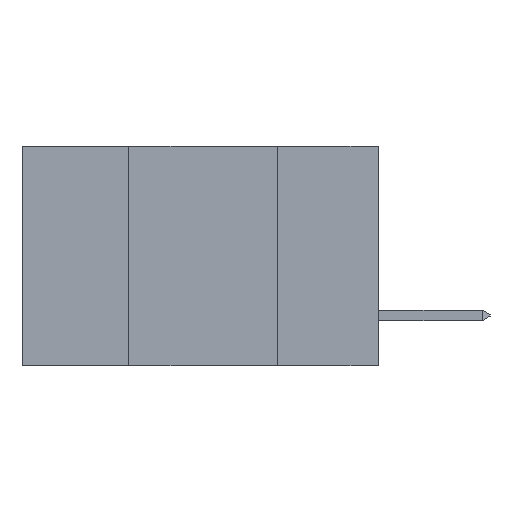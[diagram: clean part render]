
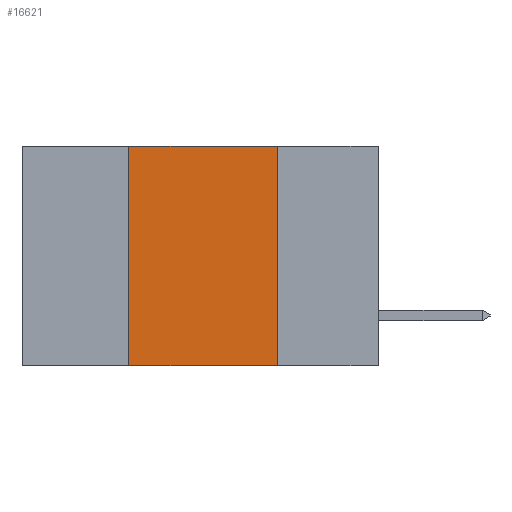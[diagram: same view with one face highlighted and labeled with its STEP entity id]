
A CAD part, left-side view. The second image highlights one B-rep face of the part: STEP entity #16621.
In plain terms, the highlighted planar face has unit normal (-1, 0, 0).
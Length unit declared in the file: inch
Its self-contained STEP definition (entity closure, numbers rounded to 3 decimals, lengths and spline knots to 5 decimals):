
#83 = CARTESIAN_POINT ( 'NONE',  ( 0., 0.42, 0. ) ) ;
#1425 = CARTESIAN_POINT ( 'NONE',  ( 0., 0.6, 0. ) ) ;
#1878 = LINE ( 'NONE', #16926, #7051 ) ;
#2397 = LINE ( 'NONE', #1425, #13970 ) ;
#3669 = DIRECTION ( 'NONE',  ( 0., -1., 0. ) ) ;
#4188 = VERTEX_POINT ( 'NONE', #4534 ) ;
#4217 = LINE ( 'NONE', #25350, #27465 ) ;
#4332 = VERTEX_POINT ( 'NONE', #6952 ) ;
#4534 = CARTESIAN_POINT ( 'NONE',  ( 0., 0.17, -0.37 ) ) ;
#6100 = DIRECTION ( 'NONE',  ( 0., 0., 1. ) ) ;
#6738 = DIRECTION ( 'NONE',  ( 0., 0., -1. ) ) ;
#6952 = CARTESIAN_POINT ( 'NONE',  ( 0., 0.17, 0. ) ) ;
#7051 = VECTOR ( 'NONE', #6100, 39.37008 ) ;
#7113 = CARTESIAN_POINT ( 'NONE',  ( 0., 0.42, -0.37 ) ) ;
#7771 = VECTOR ( 'NONE', #12759, 39.37008 ) ;
#8272 = ORIENTED_EDGE ( 'NONE', *, *, #16492, .F. ) ;
#9419 = EDGE_CURVE ( 'NONE', #14045, #4332, #2397, .T. ) ;
#12649 = ORIENTED_EDGE ( 'NONE', *, *, #9419, .F. ) ;
#12759 = DIRECTION ( 'NONE',  ( 0., 0., -1. ) ) ;
#12953 = EDGE_LOOP ( 'NONE', ( #8272, #12649, #23379, #15118 ) ) ;
#13136 = CARTESIAN_POINT ( 'NONE',  ( 0., 0.6, 0. ) ) ;
#13970 = VECTOR ( 'NONE', #3669, 39.37008 ) ;
#14045 = VERTEX_POINT ( 'NONE', #83 ) ;
#15118 = ORIENTED_EDGE ( 'NONE', *, *, #18301, .T. ) ;
#16492 = EDGE_CURVE ( 'NONE', #4332, #4188, #24536, .T. ) ;
#16621 = ADVANCED_FACE ( 'NONE', ( #21077 ), #19676, .F. ) ;
#16926 = CARTESIAN_POINT ( 'NONE',  ( 0., 0.42, 0. ) ) ;
#18301 = EDGE_CURVE ( 'NONE', #22115, #4188, #4217, .T. ) ;
#19498 = AXIS2_PLACEMENT_3D ( 'NONE', #13136, #19767, #6738 ) ;
#19676 = PLANE ( 'NONE',  #19498 ) ;
#19767 = DIRECTION ( 'NONE',  ( 1., 0., 0. ) ) ;
#21077 = FACE_OUTER_BOUND ( 'NONE', #12953, .T. ) ;
#22115 = VERTEX_POINT ( 'NONE', #7113 ) ;
#23064 = DIRECTION ( 'NONE',  ( 0., -1., 0. ) ) ;
#23126 = EDGE_CURVE ( 'NONE', #22115, #14045, #1878, .T. ) ;
#23379 = ORIENTED_EDGE ( 'NONE', *, *, #23126, .F. ) ;
#24536 = LINE ( 'NONE', #25936, #7771 ) ;
#25350 = CARTESIAN_POINT ( 'NONE',  ( 0., 0.6, -0.37 ) ) ;
#25936 = CARTESIAN_POINT ( 'NONE',  ( 0., 0.17, 0. ) ) ;
#27465 = VECTOR ( 'NONE', #23064, 39.37008 ) ;
